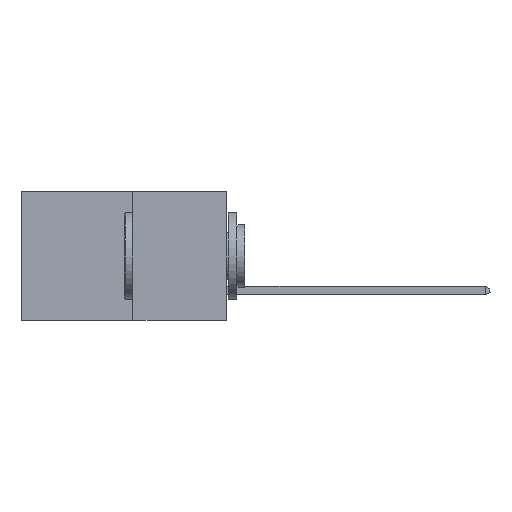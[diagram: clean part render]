
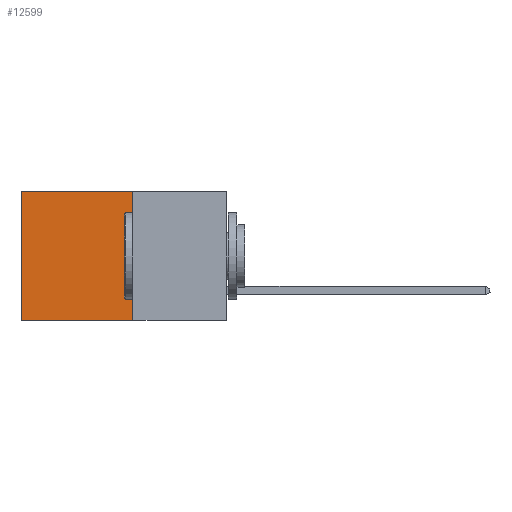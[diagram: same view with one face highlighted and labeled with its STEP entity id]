
A CAD part, left-side view. The second image highlights one B-rep face of the part: STEP entity #12599.
In plain terms, the highlighted planar face has unit normal (-1, 0, 0).
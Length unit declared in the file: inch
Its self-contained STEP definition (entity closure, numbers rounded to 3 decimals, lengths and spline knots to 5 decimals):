
#238 = FACE_OUTER_BOUND ( 'NONE', #6643, .T. ) ;
#1073 = CARTESIAN_POINT ( 'NONE',  ( 0.277, 0.27, 0. ) ) ;
#2411 = CARTESIAN_POINT ( 'NONE',  ( 0.277, 0.27, -0.37 ) ) ;
#2591 = ORIENTED_EDGE ( 'NONE', *, *, #7468, .T. ) ;
#2863 = LINE ( 'NONE', #10166, #19282 ) ;
#2890 = VERTEX_POINT ( 'NONE', #1073 ) ;
#3051 = VERTEX_POINT ( 'NONE', #19109 ) ;
#3292 = EDGE_CURVE ( 'NONE', #3051, #3309, #19867, .T. ) ;
#3309 = VERTEX_POINT ( 'NONE', #7519 ) ;
#3913 = VECTOR ( 'NONE', #14467, 39.37008 ) ;
#4076 = DIRECTION ( 'NONE',  ( 0., 0., -1. ) ) ;
#5128 = DIRECTION ( 'NONE',  ( 0., 1., 0. ) ) ;
#5361 = CARTESIAN_POINT ( 'NONE',  ( 0.277, 0.27, -0.37 ) ) ;
#6543 = VECTOR ( 'NONE', #10336, 39.37008 ) ;
#6643 = EDGE_LOOP ( 'NONE', ( #15217, #7928, #18235, #2591 ) ) ;
#7468 = EDGE_CURVE ( 'NONE', #2890, #19788, #2863, .T. ) ;
#7519 = CARTESIAN_POINT ( 'NONE',  ( 0.277, 0.59, -0.37 ) ) ;
#7928 = ORIENTED_EDGE ( 'NONE', *, *, #3292, .F. ) ;
#9409 = CARTESIAN_POINT ( 'NONE',  ( 0.277, 0.59, -0.37 ) ) ;
#10044 = DIRECTION ( 'NONE',  ( 0., 1., 0. ) ) ;
#10166 = CARTESIAN_POINT ( 'NONE',  ( 0.277, 0.27, 0. ) ) ;
#10336 = DIRECTION ( 'NONE',  ( 0., 0., -1. ) ) ;
#10551 = EDGE_CURVE ( 'NONE', #2890, #3051, #19178, .T. ) ;
#11080 = CARTESIAN_POINT ( 'NONE',  ( 0.277, 0.59, 0. ) ) ;
#12083 = VECTOR ( 'NONE', #5128, 39.37008 ) ;
#12134 = PLANE ( 'NONE',  #14166 ) ;
#12599 = ADVANCED_FACE ( 'NONE', ( #238 ), #12134, .F. ) ;
#12817 = EDGE_CURVE ( 'NONE', #19788, #3309, #17171, .T. ) ;
#13707 = DIRECTION ( 'NONE',  ( 1., 0., 0. ) ) ;
#14166 = AXIS2_PLACEMENT_3D ( 'NONE', #2411, #13707, #4076 ) ;
#14467 = DIRECTION ( 'NONE',  ( 0., 0., -1. ) ) ;
#15217 = ORIENTED_EDGE ( 'NONE', *, *, #12817, .T. ) ;
#17171 = LINE ( 'NONE', #9409, #3913 ) ;
#18235 = ORIENTED_EDGE ( 'NONE', *, *, #10551, .F. ) ;
#19109 = CARTESIAN_POINT ( 'NONE',  ( 0.277, 0.27, -0.37 ) ) ;
#19178 = LINE ( 'NONE', #19621, #6543 ) ;
#19282 = VECTOR ( 'NONE', #10044, 39.37008 ) ;
#19621 = CARTESIAN_POINT ( 'NONE',  ( 0.277, 0.27, -0.37 ) ) ;
#19788 = VERTEX_POINT ( 'NONE', #11080 ) ;
#19867 = LINE ( 'NONE', #5361, #12083 ) ;
